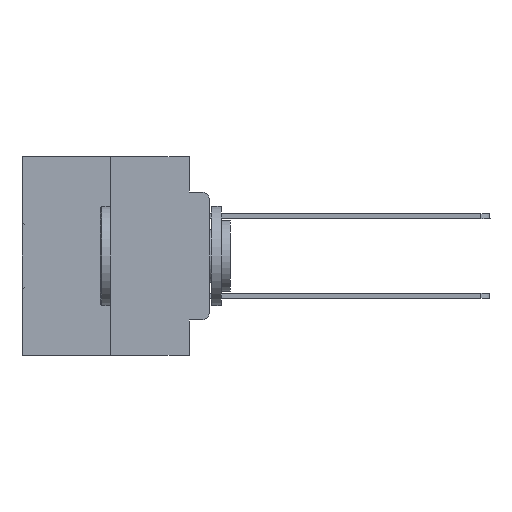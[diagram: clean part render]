
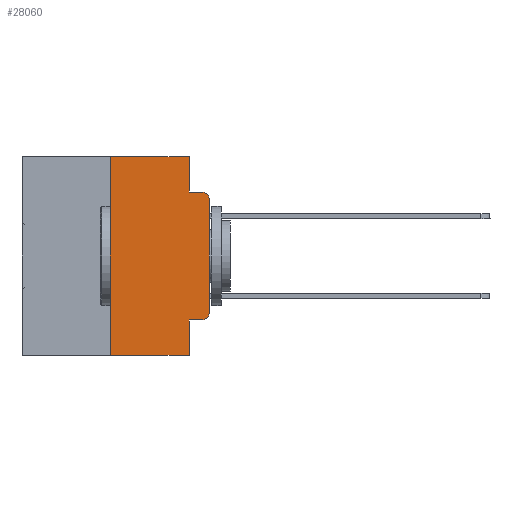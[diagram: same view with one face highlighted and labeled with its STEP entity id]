
A CAD part, left-side view. The second image highlights one B-rep face of the part: STEP entity #28060.
In plain terms, the highlighted planar face has unit normal (-1, 0, 0).
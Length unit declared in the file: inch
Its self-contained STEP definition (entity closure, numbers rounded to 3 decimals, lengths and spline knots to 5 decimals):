
#655 = CARTESIAN_POINT ( 'NONE',  ( 0., 0.051, -0.4115 ) ) ;
#839 = CARTESIAN_POINT ( 'NONE',  ( 0., 0.051, 0. ) ) ;
#964 = CIRCLE ( 'NONE', #24610, 0.02 ) ;
#1249 = EDGE_CURVE ( 'NONE', #5510, #15208, #15695, .T. ) ;
#1452 = CARTESIAN_POINT ( 'NONE',  ( 0., 0.02, -0.0885 ) ) ;
#2661 = CARTESIAN_POINT ( 'NONE',  ( 0., 0.02, -0.1085 ) ) ;
#2841 = CARTESIAN_POINT ( 'NONE',  ( 0., 0.473, 0. ) ) ;
#2987 = LINE ( 'NONE', #16956, #9121 ) ;
#3100 = DIRECTION ( 'NONE',  ( 0., 0., -1. ) ) ;
#3378 = CARTESIAN_POINT ( 'NONE',  ( 0., 0.051, -0.0885 ) ) ;
#3449 = DIRECTION ( 'NONE',  ( -1., 0., 0. ) ) ;
#3749 = CARTESIAN_POINT ( 'NONE',  ( 0., 0.473, 0. ) ) ;
#4755 = LINE ( 'NONE', #12167, #21418 ) ;
#5217 = AXIS2_PLACEMENT_3D ( 'NONE', #15289, #18006, #17565 ) ;
#5240 = ORIENTED_EDGE ( 'NONE', *, *, #18636, .T. ) ;
#5510 = VERTEX_POINT ( 'NONE', #20438 ) ;
#6074 = CARTESIAN_POINT ( 'NONE',  ( 0., 0.051, -0.0885 ) ) ;
#6363 = DIRECTION ( 'NONE',  ( 0., 0., -1. ) ) ;
#6533 = DIRECTION ( 'NONE',  ( 0., -1., 0. ) ) ;
#7113 = CARTESIAN_POINT ( 'NONE',  ( 0., 0., 0. ) ) ;
#7210 = DIRECTION ( 'NONE',  ( 0., 0., 1. ) ) ;
#7458 = EDGE_CURVE ( 'NONE', #19927, #14980, #16734, .T. ) ;
#8104 = LINE ( 'NONE', #839, #23638 ) ;
#8151 = FACE_OUTER_BOUND ( 'NONE', #27295, .T. ) ;
#8671 = ORIENTED_EDGE ( 'NONE', *, *, #31087, .T. ) ;
#8937 = CARTESIAN_POINT ( 'NONE',  ( 0., 0.051, 0. ) ) ;
#9011 = LINE ( 'NONE', #28297, #25746 ) ;
#9121 = VECTOR ( 'NONE', #22081, 39.37008 ) ;
#9671 = CARTESIAN_POINT ( 'NONE',  ( 0., 0.051, -0.4115 ) ) ;
#10180 = VECTOR ( 'NONE', #6533, 39.37008 ) ;
#10658 = ORIENTED_EDGE ( 'NONE', *, *, #17745, .T. ) ;
#12167 = CARTESIAN_POINT ( 'NONE',  ( 0., 0.473, -0.5 ) ) ;
#12220 = VERTEX_POINT ( 'NONE', #21414 ) ;
#13333 = DIRECTION ( 'NONE',  ( 0., -1., 0. ) ) ;
#13770 = DIRECTION ( 'NONE',  ( 1., 0., 0. ) ) ;
#14219 = VERTEX_POINT ( 'NONE', #24563 ) ;
#14578 = DIRECTION ( 'NONE',  ( 0., -1., 0. ) ) ;
#14980 = VERTEX_POINT ( 'NONE', #1452 ) ;
#15144 = VERTEX_POINT ( 'NONE', #32204 ) ;
#15208 = VERTEX_POINT ( 'NONE', #25142 ) ;
#15289 = CARTESIAN_POINT ( 'NONE',  ( 0., 0.02, -0.3915 ) ) ;
#15695 = LINE ( 'NONE', #7113, #22270 ) ;
#15745 = ORIENTED_EDGE ( 'NONE', *, *, #33675, .T. ) ;
#16729 = PLANE ( 'NONE',  #22640 ) ;
#16734 = LINE ( 'NONE', #6074, #10180 ) ;
#16956 = CARTESIAN_POINT ( 'NONE',  ( 0., 0.051, 0. ) ) ;
#17213 = ORIENTED_EDGE ( 'NONE', *, *, #1249, .T. ) ;
#17397 = EDGE_CURVE ( 'NONE', #20934, #28690, #30895, .T. ) ;
#17449 = VERTEX_POINT ( 'NONE', #655 ) ;
#17565 = DIRECTION ( 'NONE',  ( 0., 0., -1. ) ) ;
#17745 = EDGE_CURVE ( 'NONE', #12220, #15144, #4755, .T. ) ;
#18006 = DIRECTION ( 'NONE',  ( -1., 0., 0. ) ) ;
#18636 = EDGE_CURVE ( 'NONE', #15208, #14980, #964, .T. ) ;
#19927 = VERTEX_POINT ( 'NONE', #3378 ) ;
#20438 = CARTESIAN_POINT ( 'NONE',  ( 0., 0., -0.3915 ) ) ;
#20934 = VERTEX_POINT ( 'NONE', #29999 ) ;
#21414 = CARTESIAN_POINT ( 'NONE',  ( 0., 0.25, -0.5 ) ) ;
#21418 = VECTOR ( 'NONE', #30658, 39.37008 ) ;
#21938 = ORIENTED_EDGE ( 'NONE', *, *, #25996, .F. ) ;
#22081 = DIRECTION ( 'NONE',  ( 0., 0., -1. ) ) ;
#22270 = VECTOR ( 'NONE', #22635, 39.37008 ) ;
#22635 = DIRECTION ( 'NONE',  ( 0., 0., 1. ) ) ;
#22640 = AXIS2_PLACEMENT_3D ( 'NONE', #3749, #13770, #6363 ) ;
#23638 = VECTOR ( 'NONE', #32093, 39.37008 ) ;
#24563 = CARTESIAN_POINT ( 'NONE',  ( 0., 0.02, -0.4115 ) ) ;
#24610 = AXIS2_PLACEMENT_3D ( 'NONE', #2661, #3449, #3100 ) ;
#25142 = CARTESIAN_POINT ( 'NONE',  ( 0., 0., -0.1085 ) ) ;
#25746 = VECTOR ( 'NONE', #7210, 39.37008 ) ;
#25996 = EDGE_CURVE ( 'NONE', #17449, #15144, #2987, .T. ) ;
#26110 = LINE ( 'NONE', #9671, #32207 ) ;
#26859 = ORIENTED_EDGE ( 'NONE', *, *, #28579, .F. ) ;
#27295 = EDGE_LOOP ( 'NONE', ( #17213, #5240, #29899, #26859, #32947, #27886, #10658, #21938, #8671, #15745 ) ) ;
#27886 = ORIENTED_EDGE ( 'NONE', *, *, #30502, .F. ) ;
#27962 = CIRCLE ( 'NONE', #5217, 0.02 ) ;
#28060 = ADVANCED_FACE ( 'NONE', ( #8151 ), #16729, .F. ) ;
#28297 = CARTESIAN_POINT ( 'NONE',  ( 0., 0.25, 0. ) ) ;
#28579 = EDGE_CURVE ( 'NONE', #28690, #19927, #8104, .T. ) ;
#28690 = VERTEX_POINT ( 'NONE', #8937 ) ;
#29239 = VECTOR ( 'NONE', #13333, 39.37008 ) ;
#29899 = ORIENTED_EDGE ( 'NONE', *, *, #7458, .F. ) ;
#29999 = CARTESIAN_POINT ( 'NONE',  ( 0., 0.25, 0. ) ) ;
#30502 = EDGE_CURVE ( 'NONE', #12220, #20934, #9011, .T. ) ;
#30658 = DIRECTION ( 'NONE',  ( 0., -1., 0. ) ) ;
#30895 = LINE ( 'NONE', #2841, #29239 ) ;
#31087 = EDGE_CURVE ( 'NONE', #17449, #14219, #26110, .T. ) ;
#32093 = DIRECTION ( 'NONE',  ( 0., 0., -1. ) ) ;
#32204 = CARTESIAN_POINT ( 'NONE',  ( 0., 0.051, -0.5 ) ) ;
#32207 = VECTOR ( 'NONE', #14578, 39.37008 ) ;
#32947 = ORIENTED_EDGE ( 'NONE', *, *, #17397, .F. ) ;
#33675 = EDGE_CURVE ( 'NONE', #14219, #5510, #27962, .T. ) ;
